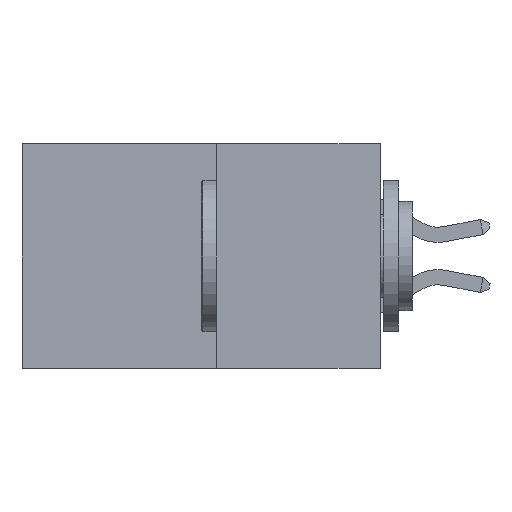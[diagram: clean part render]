
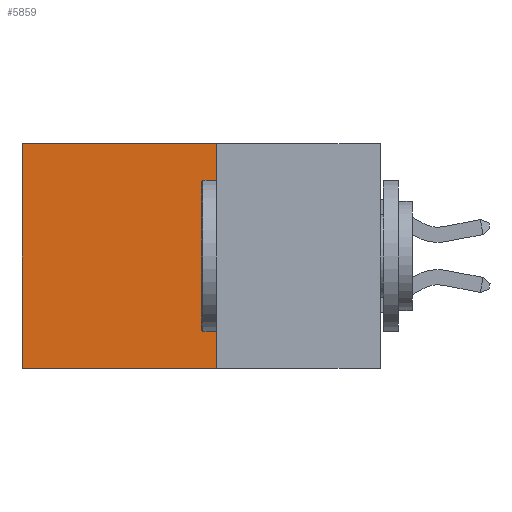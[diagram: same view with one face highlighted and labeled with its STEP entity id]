
A CAD part, left-side view. The second image highlights one B-rep face of the part: STEP entity #5859.
In plain terms, the highlighted planar face has unit normal (-1, 0, 0).
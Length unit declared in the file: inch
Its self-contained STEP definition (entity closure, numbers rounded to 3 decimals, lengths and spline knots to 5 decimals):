
#1166 = VERTEX_POINT ( 'NONE', #25441 ) ;
#2286 = DIRECTION ( 'NONE',  ( 0., 1., 0. ) ) ;
#2501 = FACE_OUTER_BOUND ( 'NONE', #27820, .T. ) ;
#2710 = ORIENTED_EDGE ( 'NONE', *, *, #18789, .F. ) ;
#3413 = EDGE_CURVE ( 'NONE', #30076, #27958, #23458, .T. ) ;
#4546 = EDGE_CURVE ( 'NONE', #27958, #1166, #24186, .T. ) ;
#5587 = DIRECTION ( 'NONE',  ( 0., 0., -1. ) ) ;
#5797 = DIRECTION ( 'NONE',  ( 1., 0., 0. ) ) ;
#5859 = ADVANCED_FACE ( 'NONE', ( #2501 ), #6357, .F. ) ;
#5999 = CARTESIAN_POINT ( 'NONE',  ( 0.277, 0.27, 0. ) ) ;
#6200 = CARTESIAN_POINT ( 'NONE',  ( 0.277, 0.27, -0.37 ) ) ;
#6357 = PLANE ( 'NONE',  #18612 ) ;
#8213 = ORIENTED_EDGE ( 'NONE', *, *, #31222, .F. ) ;
#8908 = VECTOR ( 'NONE', #28818, 39.37008 ) ;
#8910 = CARTESIAN_POINT ( 'NONE',  ( 0.277, 0.59, -0.37 ) ) ;
#9714 = CARTESIAN_POINT ( 'NONE',  ( 0.277, 0.59, 0. ) ) ;
#10181 = VERTEX_POINT ( 'NONE', #26883 ) ;
#11208 = VECTOR ( 'NONE', #31628, 39.37008 ) ;
#11436 = ORIENTED_EDGE ( 'NONE', *, *, #3413, .T. ) ;
#11900 = CARTESIAN_POINT ( 'NONE',  ( 0.277, 0.27, -0.37 ) ) ;
#14092 = VECTOR ( 'NONE', #16803, 39.37008 ) ;
#14148 = CARTESIAN_POINT ( 'NONE',  ( 0.277, 0.27, -0.37 ) ) ;
#16803 = DIRECTION ( 'NONE',  ( 0., 0., -1. ) ) ;
#16851 = ORIENTED_EDGE ( 'NONE', *, *, #4546, .T. ) ;
#16960 = VECTOR ( 'NONE', #2286, 39.37008 ) ;
#18612 = AXIS2_PLACEMENT_3D ( 'NONE', #6200, #5797, #5587 ) ;
#18789 = EDGE_CURVE ( 'NONE', #30076, #10181, #27086, .T. ) ;
#23458 = LINE ( 'NONE', #5999, #16960 ) ;
#24186 = LINE ( 'NONE', #8910, #11208 ) ;
#25441 = CARTESIAN_POINT ( 'NONE',  ( 0.277, 0.59, -0.37 ) ) ;
#26883 = CARTESIAN_POINT ( 'NONE',  ( 0.277, 0.27, -0.37 ) ) ;
#27086 = LINE ( 'NONE', #11900, #14092 ) ;
#27820 = EDGE_LOOP ( 'NONE', ( #16851, #8213, #2710, #11436 ) ) ;
#27958 = VERTEX_POINT ( 'NONE', #9714 ) ;
#28466 = LINE ( 'NONE', #14148, #8908 ) ;
#28818 = DIRECTION ( 'NONE',  ( 0., 1., 0. ) ) ;
#29440 = CARTESIAN_POINT ( 'NONE',  ( 0.277, 0.27, 0. ) ) ;
#30076 = VERTEX_POINT ( 'NONE', #29440 ) ;
#31222 = EDGE_CURVE ( 'NONE', #10181, #1166, #28466, .T. ) ;
#31628 = DIRECTION ( 'NONE',  ( 0., 0., -1. ) ) ;
